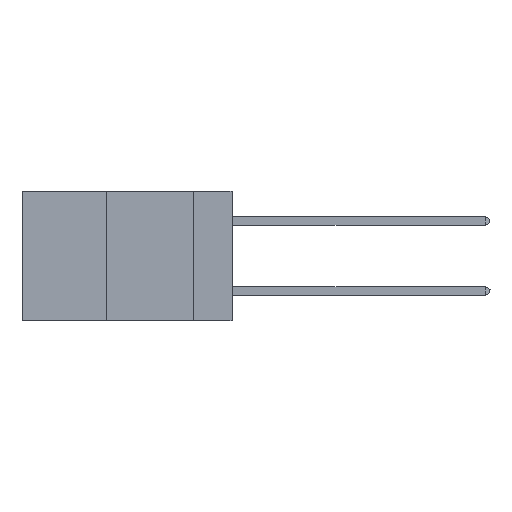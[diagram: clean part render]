
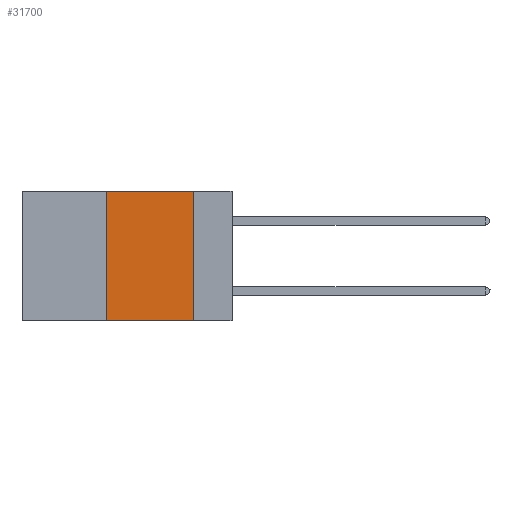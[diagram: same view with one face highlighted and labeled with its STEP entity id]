
A CAD part, left-side view. The second image highlights one B-rep face of the part: STEP entity #31700.
In plain terms, the highlighted planar face has unit normal (-1, 0, 0).
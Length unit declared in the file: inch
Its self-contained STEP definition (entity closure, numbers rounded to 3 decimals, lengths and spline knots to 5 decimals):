
#1666 = CARTESIAN_POINT ( 'NONE',  ( 0., 0.6, -0.37 ) ) ;
#2126 = LINE ( 'NONE', #12366, #32929 ) ;
#2993 = EDGE_CURVE ( 'NONE', #30016, #25823, #2126, .T. ) ;
#3302 = DIRECTION ( 'NONE',  ( 0., 0., -1. ) ) ;
#4364 = EDGE_CURVE ( 'NONE', #25823, #12503, #7633, .T. ) ;
#6198 = CARTESIAN_POINT ( 'NONE',  ( 0., 0.36, -0.37 ) ) ;
#6210 = VERTEX_POINT ( 'NONE', #7042 ) ;
#7042 = CARTESIAN_POINT ( 'NONE',  ( 0., 0.11, -0.37 ) ) ;
#7541 = LINE ( 'NONE', #14212, #11424 ) ;
#7633 = LINE ( 'NONE', #17592, #33282 ) ;
#9472 = DIRECTION ( 'NONE',  ( 0., -1., 0. ) ) ;
#10857 = CARTESIAN_POINT ( 'NONE',  ( 0., 0.36, 0. ) ) ;
#11424 = VECTOR ( 'NONE', #3302, 39.37008 ) ;
#12366 = CARTESIAN_POINT ( 'NONE',  ( 0., 0.36, 0. ) ) ;
#12503 = VERTEX_POINT ( 'NONE', #24138 ) ;
#13938 = VECTOR ( 'NONE', #23288, 39.37008 ) ;
#14212 = CARTESIAN_POINT ( 'NONE',  ( 0., 0.11, 0. ) ) ;
#16835 = ORIENTED_EDGE ( 'NONE', *, *, #30685, .F. ) ;
#17592 = CARTESIAN_POINT ( 'NONE',  ( 0., 0.6, 0. ) ) ;
#20810 = DIRECTION ( 'NONE',  ( 0., 0., 1. ) ) ;
#22121 = ORIENTED_EDGE ( 'NONE', *, *, #23451, .T. ) ;
#22827 = FACE_OUTER_BOUND ( 'NONE', #24450, .T. ) ;
#23288 = DIRECTION ( 'NONE',  ( 0., -1., 0. ) ) ;
#23451 = EDGE_CURVE ( 'NONE', #30016, #6210, #28865, .T. ) ;
#24138 = CARTESIAN_POINT ( 'NONE',  ( 0., 0.11, 0. ) ) ;
#24450 = EDGE_LOOP ( 'NONE', ( #16835, #27638, #28787, #22121 ) ) ;
#25823 = VERTEX_POINT ( 'NONE', #10857 ) ;
#26513 = PLANE ( 'NONE',  #32641 ) ;
#27638 = ORIENTED_EDGE ( 'NONE', *, *, #4364, .F. ) ;
#28787 = ORIENTED_EDGE ( 'NONE', *, *, #2993, .F. ) ;
#28865 = LINE ( 'NONE', #1666, #13938 ) ;
#29228 = DIRECTION ( 'NONE',  ( 0., 0., -1. ) ) ;
#30016 = VERTEX_POINT ( 'NONE', #6198 ) ;
#30685 = EDGE_CURVE ( 'NONE', #12503, #6210, #7541, .T. ) ;
#31700 = ADVANCED_FACE ( 'NONE', ( #22827 ), #26513, .F. ) ;
#32340 = DIRECTION ( 'NONE',  ( 1., 0., 0. ) ) ;
#32641 = AXIS2_PLACEMENT_3D ( 'NONE', #34970, #32340, #29228 ) ;
#32929 = VECTOR ( 'NONE', #20810, 39.37008 ) ;
#33282 = VECTOR ( 'NONE', #9472, 39.37008 ) ;
#34970 = CARTESIAN_POINT ( 'NONE',  ( 0., 0.6, 0. ) ) ;
